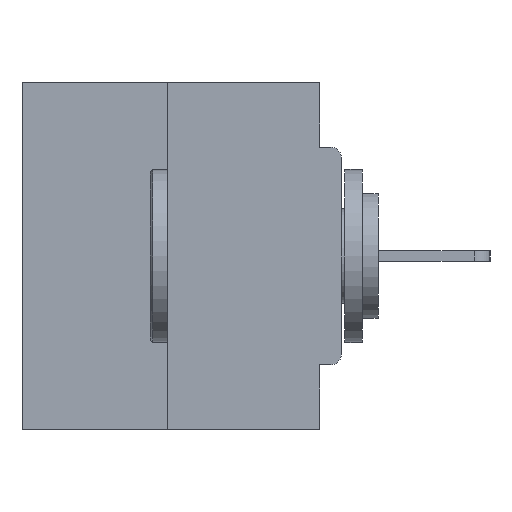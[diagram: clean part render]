
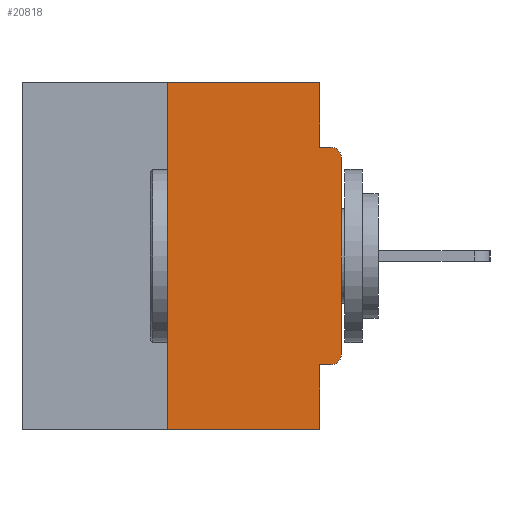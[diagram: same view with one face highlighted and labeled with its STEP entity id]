
A CAD part, left-side view. The second image highlights one B-rep face of the part: STEP entity #20818.
In plain terms, the highlighted planar face has unit normal (-1, 0, 0).
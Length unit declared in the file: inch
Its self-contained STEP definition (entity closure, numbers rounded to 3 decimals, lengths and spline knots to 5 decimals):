
#379 = EDGE_CURVE ( 'NONE', #9936, #10009, #5783, .T. ) ;
#694 = VECTOR ( 'NONE', #30550, 39.37008 ) ;
#725 = ORIENTED_EDGE ( 'NONE', *, *, #4306, .T. ) ;
#887 = CARTESIAN_POINT ( 'NONE',  ( 0., 0.031, -0.0935 ) ) ;
#1625 = DIRECTION ( 'NONE',  ( 0., 0., 1. ) ) ;
#1685 = EDGE_CURVE ( 'NONE', #24703, #29714, #21631, .T. ) ;
#1721 = CARTESIAN_POINT ( 'NONE',  ( 0., 0.25, -0.5 ) ) ;
#2970 = ORIENTED_EDGE ( 'NONE', *, *, #30201, .F. ) ;
#3117 = CARTESIAN_POINT ( 'NONE',  ( 0., 0., -0.4065 ) ) ;
#4300 = VERTEX_POINT ( 'NONE', #887 ) ;
#4306 = EDGE_CURVE ( 'NONE', #17418, #13932, #7354, .T. ) ;
#4308 = FACE_OUTER_BOUND ( 'NONE', #11790, .T. ) ;
#4427 = VECTOR ( 'NONE', #18834, 39.37008 ) ;
#4929 = VECTOR ( 'NONE', #22233, 39.37008 ) ;
#5124 = EDGE_CURVE ( 'NONE', #5884, #25148, #18151, .T. ) ;
#5783 = CIRCLE ( 'NONE', #12008, 0.015 ) ;
#5884 = VERTEX_POINT ( 'NONE', #10231 ) ;
#6848 = CARTESIAN_POINT ( 'NONE',  ( 0., 0., 0. ) ) ;
#7017 = CARTESIAN_POINT ( 'NONE',  ( 0., 0.031, -0.5 ) ) ;
#7354 = LINE ( 'NONE', #10830, #22855 ) ;
#8768 = CARTESIAN_POINT ( 'NONE',  ( 0., 0.015, -0.1085 ) ) ;
#8834 = DIRECTION ( 'NONE',  ( 0., 0., -1. ) ) ;
#9405 = LINE ( 'NONE', #6848, #12090 ) ;
#9860 = EDGE_CURVE ( 'NONE', #19155, #9936, #9405, .T. ) ;
#9936 = VERTEX_POINT ( 'NONE', #13352 ) ;
#9986 = CARTESIAN_POINT ( 'NONE',  ( 0., 0., -0.3915 ) ) ;
#9994 = LINE ( 'NONE', #11354, #30966 ) ;
#9998 = EDGE_CURVE ( 'NONE', #5884, #19155, #15966, .T. ) ;
#10009 = VERTEX_POINT ( 'NONE', #21237 ) ;
#10231 = CARTESIAN_POINT ( 'NONE',  ( 0., 0.015, -0.4065 ) ) ;
#10827 = CARTESIAN_POINT ( 'NONE',  ( 0., 0.015, -0.3915 ) ) ;
#10830 = CARTESIAN_POINT ( 'NONE',  ( 0., 0.46, -0.5 ) ) ;
#11033 = LINE ( 'NONE', #16457, #4427 ) ;
#11106 = PLANE ( 'NONE',  #23855 ) ;
#11260 = DIRECTION ( 'NONE',  ( 0., 0., -1. ) ) ;
#11354 = CARTESIAN_POINT ( 'NONE',  ( 0., 0.25, 0. ) ) ;
#11790 = EDGE_LOOP ( 'NONE', ( #29409, #24293, #725, #12718, #30867, #14955, #11913, #28121, #22137, #2970 ) ) ;
#11913 = ORIENTED_EDGE ( 'NONE', *, *, #9860, .T. ) ;
#12008 = AXIS2_PLACEMENT_3D ( 'NONE', #8768, #26117, #11260 ) ;
#12090 = VECTOR ( 'NONE', #16415, 39.37008 ) ;
#12718 = ORIENTED_EDGE ( 'NONE', *, *, #22086, .F. ) ;
#13119 = EDGE_CURVE ( 'NONE', #4300, #10009, #25659, .T. ) ;
#13352 = CARTESIAN_POINT ( 'NONE',  ( 0., 0., -0.1085 ) ) ;
#13932 = VERTEX_POINT ( 'NONE', #21172 ) ;
#14422 = DIRECTION ( 'NONE',  ( 0., 0., -1. ) ) ;
#14955 = ORIENTED_EDGE ( 'NONE', *, *, #9998, .T. ) ;
#15824 = DIRECTION ( 'NONE',  ( -1., 0., 0. ) ) ;
#15966 = CIRCLE ( 'NONE', #20759, 0.015 ) ;
#16415 = DIRECTION ( 'NONE',  ( 0., 0., 1. ) ) ;
#16457 = CARTESIAN_POINT ( 'NONE',  ( 0., 0.031, 0. ) ) ;
#17418 = VERTEX_POINT ( 'NONE', #1721 ) ;
#18151 = LINE ( 'NONE', #3117, #694 ) ;
#18333 = DIRECTION ( 'NONE',  ( 0., 0., -1. ) ) ;
#18814 = CARTESIAN_POINT ( 'NONE',  ( 0., 0.46, 0. ) ) ;
#18834 = DIRECTION ( 'NONE',  ( 0., 0., -1. ) ) ;
#19155 = VERTEX_POINT ( 'NONE', #9986 ) ;
#20739 = CARTESIAN_POINT ( 'NONE',  ( 0., 0.031, -0.4065 ) ) ;
#20759 = AXIS2_PLACEMENT_3D ( 'NONE', #10827, #15824, #18333 ) ;
#20818 = ADVANCED_FACE ( 'NONE', ( #4308 ), #11106, .F. ) ;
#21172 = CARTESIAN_POINT ( 'NONE',  ( 0., 0.031, -0.5 ) ) ;
#21237 = CARTESIAN_POINT ( 'NONE',  ( 0., 0.015, -0.0935 ) ) ;
#21309 = DIRECTION ( 'NONE',  ( 1., 0., 0. ) ) ;
#21631 = LINE ( 'NONE', #26911, #4929 ) ;
#21954 = CARTESIAN_POINT ( 'NONE',  ( 0., 0.25, 0. ) ) ;
#22086 = EDGE_CURVE ( 'NONE', #25148, #13932, #31394, .T. ) ;
#22137 = ORIENTED_EDGE ( 'NONE', *, *, #13119, .F. ) ;
#22233 = DIRECTION ( 'NONE',  ( 0., -1., 0. ) ) ;
#22855 = VECTOR ( 'NONE', #30574, 39.37008 ) ;
#23855 = AXIS2_PLACEMENT_3D ( 'NONE', #18814, #21309, #8834 ) ;
#24289 = EDGE_CURVE ( 'NONE', #17418, #24703, #9994, .T. ) ;
#24293 = ORIENTED_EDGE ( 'NONE', *, *, #24289, .F. ) ;
#24703 = VERTEX_POINT ( 'NONE', #21954 ) ;
#25148 = VERTEX_POINT ( 'NONE', #20739 ) ;
#25288 = VECTOR ( 'NONE', #30658, 39.37008 ) ;
#25659 = LINE ( 'NONE', #28061, #25288 ) ;
#26117 = DIRECTION ( 'NONE',  ( -1., 0., 0. ) ) ;
#26911 = CARTESIAN_POINT ( 'NONE',  ( 0., 0.46, 0. ) ) ;
#28061 = CARTESIAN_POINT ( 'NONE',  ( 0., 0., -0.0935 ) ) ;
#28121 = ORIENTED_EDGE ( 'NONE', *, *, #379, .T. ) ;
#28271 = VECTOR ( 'NONE', #14422, 39.37008 ) ;
#28769 = CARTESIAN_POINT ( 'NONE',  ( 0., 0.031, 0. ) ) ;
#29409 = ORIENTED_EDGE ( 'NONE', *, *, #1685, .F. ) ;
#29714 = VERTEX_POINT ( 'NONE', #28769 ) ;
#30201 = EDGE_CURVE ( 'NONE', #29714, #4300, #11033, .T. ) ;
#30550 = DIRECTION ( 'NONE',  ( 0., 1., 0. ) ) ;
#30574 = DIRECTION ( 'NONE',  ( 0., -1., 0. ) ) ;
#30658 = DIRECTION ( 'NONE',  ( 0., -1., 0. ) ) ;
#30867 = ORIENTED_EDGE ( 'NONE', *, *, #5124, .F. ) ;
#30966 = VECTOR ( 'NONE', #1625, 39.37008 ) ;
#31394 = LINE ( 'NONE', #7017, #28271 ) ;
